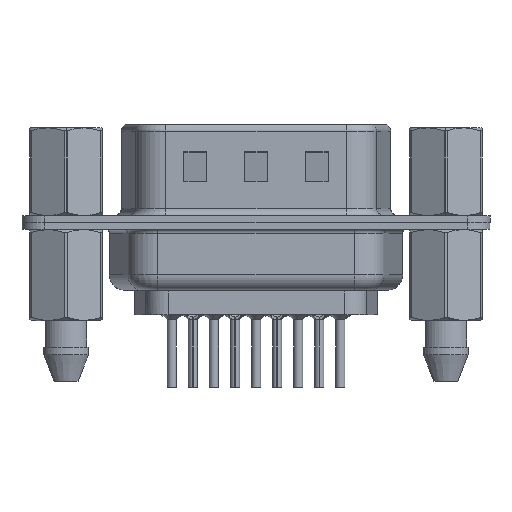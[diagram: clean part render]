
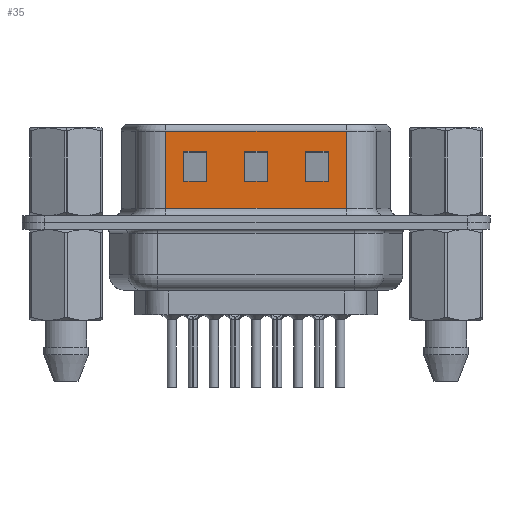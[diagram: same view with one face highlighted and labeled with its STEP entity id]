
A CAD part, front view. The second image highlights one B-rep face of the part: STEP entity #35.
In plain terms, the highlighted planar face has unit normal (0, -1, 0).
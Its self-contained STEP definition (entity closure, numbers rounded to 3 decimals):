
#35 = ADVANCED_FACE ( 'NONE', ( #11697, #9576, #15537, #21019 ), #5979, .F. ) ;
#345 = EDGE_CURVE ( 'NONE', #15712, #1332, #19746, .T. ) ;
#580 = CARTESIAN_POINT ( 'NONE',  ( 17.245, -4.58, 4.705 ) ) ;
#1199 = ORIENTED_EDGE ( 'NONE', *, *, #8510, .T. ) ;
#1276 = EDGE_CURVE ( 'NONE', #15599, #18851, #21878, .T. ) ;
#1332 = VERTEX_POINT ( 'NONE', #3724 ) ;
#1582 = LINE ( 'NONE', #9152, #1627 ) ;
#1627 = VECTOR ( 'NONE', #1700, 1000. ) ;
#1700 = DIRECTION ( 'NONE',  ( 0., 0., -1. ) ) ;
#1907 = DIRECTION ( 'NONE',  ( 0., 0., 1. ) ) ;
#2116 = LINE ( 'NONE', #11431, #5339 ) ;
#2546 = CARTESIAN_POINT ( 'NONE',  ( 13.245, -4.58, 4.705 ) ) ;
#2564 = VERTEX_POINT ( 'NONE', #19437 ) ;
#2693 = ORIENTED_EDGE ( 'NONE', *, *, #17269, .T. ) ;
#2946 = ORIENTED_EDGE ( 'NONE', *, *, #9664, .T. ) ;
#3406 = ORIENTED_EDGE ( 'NONE', *, *, #1276, .T. ) ;
#3545 = ORIENTED_EDGE ( 'NONE', *, *, #21451, .T. ) ;
#3583 = VECTOR ( 'NONE', #21730, 1000. ) ;
#3724 = CARTESIAN_POINT ( 'NONE',  ( 17.245, -4.58, 2.705 ) ) ;
#3928 = DIRECTION ( 'NONE',  ( -1., 0., 0. ) ) ;
#4011 = VECTOR ( 'NONE', #12473, 1000. ) ;
#4129 = EDGE_CURVE ( 'NONE', #1332, #22827, #16689, .T. ) ;
#4271 = CARTESIAN_POINT ( 'NONE',  ( 18.445, -4.58, 2.705 ) ) ;
#4357 = VECTOR ( 'NONE', #1907, 1000. ) ;
#4399 = LINE ( 'NONE', #4271, #22399 ) ;
#4549 = CARTESIAN_POINT ( 'NONE',  ( 14.445, -4.58, 2.705 ) ) ;
#5300 = CARTESIAN_POINT ( 'NONE',  ( 18.445, -4.58, 6.52 ) ) ;
#5339 = VECTOR ( 'NONE', #7449, 1000. ) ;
#5383 = DIRECTION ( 'NONE',  ( 1., 0., 0. ) ) ;
#5426 = CARTESIAN_POINT ( 'NONE',  ( 6.545, -4.58, 0.95 ) ) ;
#5625 = CARTESIAN_POINT ( 'NONE',  ( 15.745, -4.58, 6.52 ) ) ;
#5979 = PLANE ( 'NONE',  #18253 ) ;
#6058 = VECTOR ( 'NONE', #20196, 1000. ) ;
#6181 = VERTEX_POINT ( 'NONE', #9988 ) ;
#6225 = DIRECTION ( 'NONE',  ( 0., 1., 0. ) ) ;
#6364 = CARTESIAN_POINT ( 'NONE',  ( 11.745, -4.58, 2.705 ) ) ;
#6550 = EDGE_CURVE ( 'NONE', #19455, #15446, #18557, .T. ) ;
#6813 = VERTEX_POINT ( 'NONE', #6364 ) ;
#6836 = VECTOR ( 'NONE', #3928, 1000. ) ;
#7108 = EDGE_CURVE ( 'NONE', #24159, #17873, #2116, .T. ) ;
#7302 = VERTEX_POINT ( 'NONE', #23478 ) ;
#7363 = CARTESIAN_POINT ( 'NONE',  ( 22.445, -4.58, 4.705 ) ) ;
#7449 = DIRECTION ( 'NONE',  ( 0., 0., -1. ) ) ;
#7718 = DIRECTION ( 'NONE',  ( 1., 0., 0. ) ) ;
#7738 = ORIENTED_EDGE ( 'NONE', *, *, #23747, .T. ) ;
#7789 = ORIENTED_EDGE ( 'NONE', *, *, #6550, .T. ) ;
#8510 = EDGE_CURVE ( 'NONE', #17187, #15868, #22287, .T. ) ;
#8623 = EDGE_LOOP ( 'NONE', ( #10397, #13581, #7789, #21982 ) ) ;
#8638 = VECTOR ( 'NONE', #14993, 1000. ) ;
#9152 = CARTESIAN_POINT ( 'NONE',  ( 6.545, -4.58, 6.52 ) ) ;
#9481 = CARTESIAN_POINT ( 'NONE',  ( 11.745, -4.58, 4.705 ) ) ;
#9576 = FACE_BOUND ( 'NONE', #9626, .T. ) ;
#9626 = EDGE_LOOP ( 'NONE', ( #19219, #10854, #22366, #2946 ) ) ;
#9664 = EDGE_CURVE ( 'NONE', #6181, #15712, #20683, .T. ) ;
#9939 = VECTOR ( 'NONE', #23736, 1000. ) ;
#9988 = CARTESIAN_POINT ( 'NONE',  ( 15.745, -4.58, 4.705 ) ) ;
#10162 = CARTESIAN_POINT ( 'NONE',  ( 7.745, -4.58, 2.705 ) ) ;
#10397 = ORIENTED_EDGE ( 'NONE', *, *, #7108, .T. ) ;
#10854 = ORIENTED_EDGE ( 'NONE', *, *, #4129, .T. ) ;
#11089 = EDGE_CURVE ( 'NONE', #15446, #24159, #22106, .T. ) ;
#11091 = DIRECTION ( 'NONE',  ( -1., 0., 0. ) ) ;
#11339 = DIRECTION ( 'NONE',  ( 0., 0., 1. ) ) ;
#11431 = CARTESIAN_POINT ( 'NONE',  ( 9.245, -4.58, 6.52 ) ) ;
#11697 = FACE_BOUND ( 'NONE', #8623, .T. ) ;
#12473 = DIRECTION ( 'NONE',  ( -1., 0., 0. ) ) ;
#12653 = CARTESIAN_POINT ( 'NONE',  ( 14.445, -4.58, 4.705 ) ) ;
#12877 = CARTESIAN_POINT ( 'NONE',  ( 7.745, -4.58, 4.705 ) ) ;
#12901 = VECTOR ( 'NONE', #5383, 1000. ) ;
#13301 = EDGE_CURVE ( 'NONE', #7302, #15868, #15229, .T. ) ;
#13365 = CARTESIAN_POINT ( 'NONE',  ( 18.445, -4.58, 6.02 ) ) ;
#13581 = ORIENTED_EDGE ( 'NONE', *, *, #17981, .T. ) ;
#13686 = CARTESIAN_POINT ( 'NONE',  ( 13.245, -4.58, 2.705 ) ) ;
#13721 = DIRECTION ( 'NONE',  ( -1., 0., 0. ) ) ;
#13812 = DIRECTION ( 'NONE',  ( 0., 0., 1. ) ) ;
#14125 = LINE ( 'NONE', #4549, #4011 ) ;
#14436 = CARTESIAN_POINT ( 'NONE',  ( 13.245, -4.58, 6.52 ) ) ;
#14529 = CARTESIAN_POINT ( 'NONE',  ( 17.245, -4.58, 6.52 ) ) ;
#14993 = DIRECTION ( 'NONE',  ( 0., 0., -1. ) ) ;
#15176 = CARTESIAN_POINT ( 'NONE',  ( 18.445, -4.58, 6.52 ) ) ;
#15229 = LINE ( 'NONE', #5300, #8638 ) ;
#15265 = EDGE_LOOP ( 'NONE', ( #19423, #3545, #2693, #1199 ) ) ;
#15396 = ORIENTED_EDGE ( 'NONE', *, *, #22961, .T. ) ;
#15446 = VERTEX_POINT ( 'NONE', #12877 ) ;
#15537 = FACE_BOUND ( 'NONE', #22263, .T. ) ;
#15599 = VERTEX_POINT ( 'NONE', #2546 ) ;
#15712 = VERTEX_POINT ( 'NONE', #580 ) ;
#15752 = CARTESIAN_POINT ( 'NONE',  ( 11.745, -4.58, 6.52 ) ) ;
#15832 = CARTESIAN_POINT ( 'NONE',  ( 18.445, -4.58, 0.95 ) ) ;
#15868 = VERTEX_POINT ( 'NONE', #15832 ) ;
#16016 = CARTESIAN_POINT ( 'NONE',  ( 18.445, -4.58, 4.705 ) ) ;
#16111 = VECTOR ( 'NONE', #11091, 1000. ) ;
#16388 = EDGE_CURVE ( 'NONE', #22827, #6181, #22653, .T. ) ;
#16516 = DIRECTION ( 'NONE',  ( 1., 0., 0. ) ) ;
#16689 = LINE ( 'NONE', #16821, #16111 ) ;
#16821 = CARTESIAN_POINT ( 'NONE',  ( 22.445, -4.58, 2.705 ) ) ;
#17187 = VERTEX_POINT ( 'NONE', #5426 ) ;
#17269 = EDGE_CURVE ( 'NONE', #2564, #17187, #1582, .T. ) ;
#17873 = VERTEX_POINT ( 'NONE', #23061 ) ;
#17981 = EDGE_CURVE ( 'NONE', #17873, #19455, #14125, .T. ) ;
#18253 = AXIS2_PLACEMENT_3D ( 'NONE', #15176, #6225, #13812 ) ;
#18294 = VECTOR ( 'NONE', #7718, 1000. ) ;
#18454 = VECTOR ( 'NONE', #23346, 1000. ) ;
#18557 = LINE ( 'NONE', #20802, #21003 ) ;
#18851 = VERTEX_POINT ( 'NONE', #13686 ) ;
#19219 = ORIENTED_EDGE ( 'NONE', *, *, #345, .T. ) ;
#19423 = ORIENTED_EDGE ( 'NONE', *, *, #13301, .F. ) ;
#19437 = CARTESIAN_POINT ( 'NONE',  ( 6.545, -4.58, 6.02 ) ) ;
#19448 = EDGE_CURVE ( 'NONE', #6813, #21819, #19499, .T. ) ;
#19455 = VERTEX_POINT ( 'NONE', #10162 ) ;
#19499 = LINE ( 'NONE', #15752, #6058 ) ;
#19586 = LINE ( 'NONE', #13365, #6836 ) ;
#19746 = LINE ( 'NONE', #14529, #3583 ) ;
#20196 = DIRECTION ( 'NONE',  ( 0., 0., 1. ) ) ;
#20437 = CARTESIAN_POINT ( 'NONE',  ( 18.445, -4.58, 0.95 ) ) ;
#20683 = LINE ( 'NONE', #7363, #12901 ) ;
#20802 = CARTESIAN_POINT ( 'NONE',  ( 7.745, -4.58, 6.52 ) ) ;
#21003 = VECTOR ( 'NONE', #11339, 1000. ) ;
#21019 = FACE_OUTER_BOUND ( 'NONE', #15265, .T. ) ;
#21079 = ORIENTED_EDGE ( 'NONE', *, *, #19448, .T. ) ;
#21451 = EDGE_CURVE ( 'NONE', #7302, #2564, #19586, .T. ) ;
#21613 = LINE ( 'NONE', #16016, #18454 ) ;
#21730 = DIRECTION ( 'NONE',  ( 0., 0., -1. ) ) ;
#21819 = VERTEX_POINT ( 'NONE', #9481 ) ;
#21878 = LINE ( 'NONE', #14436, #9939 ) ;
#21982 = ORIENTED_EDGE ( 'NONE', *, *, #11089, .T. ) ;
#22106 = LINE ( 'NONE', #12653, #23412 ) ;
#22263 = EDGE_LOOP ( 'NONE', ( #7738, #3406, #15396, #21079 ) ) ;
#22287 = LINE ( 'NONE', #20437, #18294 ) ;
#22366 = ORIENTED_EDGE ( 'NONE', *, *, #16388, .T. ) ;
#22399 = VECTOR ( 'NONE', #13721, 1000. ) ;
#22653 = LINE ( 'NONE', #5625, #4357 ) ;
#22827 = VERTEX_POINT ( 'NONE', #24530 ) ;
#22961 = EDGE_CURVE ( 'NONE', #18851, #6813, #4399, .T. ) ;
#23061 = CARTESIAN_POINT ( 'NONE',  ( 9.245, -4.58, 2.705 ) ) ;
#23306 = CARTESIAN_POINT ( 'NONE',  ( 9.245, -4.58, 4.705 ) ) ;
#23346 = DIRECTION ( 'NONE',  ( 1., 0., 0. ) ) ;
#23412 = VECTOR ( 'NONE', #16516, 1000. ) ;
#23478 = CARTESIAN_POINT ( 'NONE',  ( 18.445, -4.58, 6.02 ) ) ;
#23736 = DIRECTION ( 'NONE',  ( 0., 0., -1. ) ) ;
#23747 = EDGE_CURVE ( 'NONE', #21819, #15599, #21613, .T. ) ;
#24159 = VERTEX_POINT ( 'NONE', #23306 ) ;
#24530 = CARTESIAN_POINT ( 'NONE',  ( 15.745, -4.58, 2.705 ) ) ;
